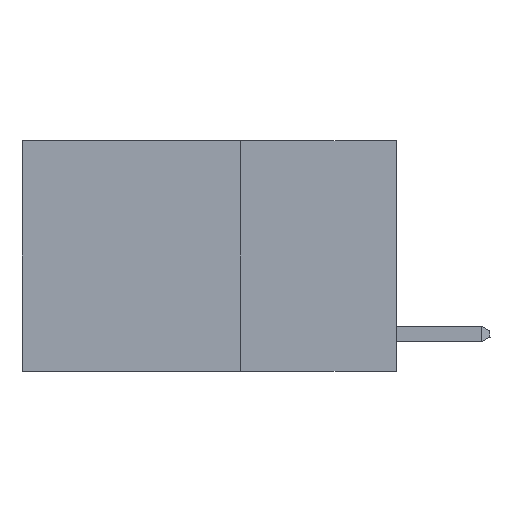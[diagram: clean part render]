
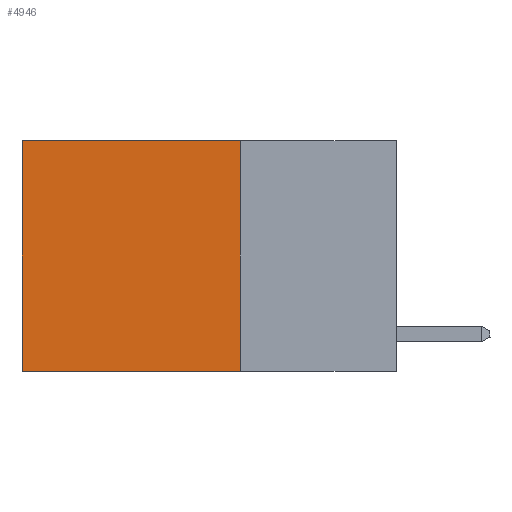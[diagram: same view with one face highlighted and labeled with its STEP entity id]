
A CAD part, left-side view. The second image highlights one B-rep face of the part: STEP entity #4946.
In plain terms, the highlighted planar face has unit normal (-1, 0, 0).
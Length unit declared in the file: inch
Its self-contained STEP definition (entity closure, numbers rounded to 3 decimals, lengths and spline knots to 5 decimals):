
#641 = LINE ( 'NONE', #1672, #12462 ) ;
#1016 = ORIENTED_EDGE ( 'NONE', *, *, #13850, .T. ) ;
#1304 = DIRECTION ( 'NONE',  ( 0., 1., 0. ) ) ;
#1390 = ORIENTED_EDGE ( 'NONE', *, *, #1830, .T. ) ;
#1672 = CARTESIAN_POINT ( 'NONE',  ( 0.2625, 0.6, 0. ) ) ;
#1830 = EDGE_CURVE ( 'NONE', #12476, #14503, #15052, .T. ) ;
#1864 = CARTESIAN_POINT ( 'NONE',  ( 0.2625, 0.6, 0. ) ) ;
#1880 = EDGE_CURVE ( 'NONE', #3887, #6609, #14695, .T. ) ;
#2609 = CARTESIAN_POINT ( 'NONE',  ( 0.2625, 0.25, -0.37 ) ) ;
#2697 = DIRECTION ( 'NONE',  ( 0., 0., -1. ) ) ;
#3112 = EDGE_LOOP ( 'NONE', ( #1016, #4233, #13528, #1390 ) ) ;
#3468 = PLANE ( 'NONE',  #6150 ) ;
#3887 = VERTEX_POINT ( 'NONE', #3915 ) ;
#3915 = CARTESIAN_POINT ( 'NONE',  ( 0.2625, 0.25, -0.37 ) ) ;
#4233 = ORIENTED_EDGE ( 'NONE', *, *, #1880, .F. ) ;
#4675 = DIRECTION ( 'NONE',  ( 1., 0., 0. ) ) ;
#4946 = ADVANCED_FACE ( 'NONE', ( #10426 ), #3468, .F. ) ;
#5145 = CARTESIAN_POINT ( 'NONE',  ( 0.2625, 0.25, 0. ) ) ;
#5855 = VECTOR ( 'NONE', #2697, 39.37008 ) ;
#6150 = AXIS2_PLACEMENT_3D ( 'NONE', #11731, #4675, #12848 ) ;
#6609 = VERTEX_POINT ( 'NONE', #9692 ) ;
#7685 = DIRECTION ( 'NONE',  ( 0., 0., -1. ) ) ;
#8481 = CARTESIAN_POINT ( 'NONE',  ( 0.2625, 0.25, 0. ) ) ;
#9007 = VECTOR ( 'NONE', #1304, 39.37008 ) ;
#9692 = CARTESIAN_POINT ( 'NONE',  ( 0.2625, 0.6, -0.37 ) ) ;
#10184 = EDGE_CURVE ( 'NONE', #12476, #3887, #14657, .T. ) ;
#10426 = FACE_OUTER_BOUND ( 'NONE', #3112, .T. ) ;
#11731 = CARTESIAN_POINT ( 'NONE',  ( 0.2625, 0.25, 0. ) ) ;
#12073 = DIRECTION ( 'NONE',  ( 0., 1., 0. ) ) ;
#12462 = VECTOR ( 'NONE', #7685, 39.37008 ) ;
#12476 = VERTEX_POINT ( 'NONE', #14401 ) ;
#12848 = DIRECTION ( 'NONE',  ( 0., 0., -1. ) ) ;
#13528 = ORIENTED_EDGE ( 'NONE', *, *, #10184, .F. ) ;
#13850 = EDGE_CURVE ( 'NONE', #14503, #6609, #641, .T. ) ;
#14016 = VECTOR ( 'NONE', #12073, 39.37008 ) ;
#14401 = CARTESIAN_POINT ( 'NONE',  ( 0.2625, 0.25, 0. ) ) ;
#14503 = VERTEX_POINT ( 'NONE', #1864 ) ;
#14657 = LINE ( 'NONE', #5145, #5855 ) ;
#14695 = LINE ( 'NONE', #2609, #14016 ) ;
#15052 = LINE ( 'NONE', #8481, #9007 ) ;
